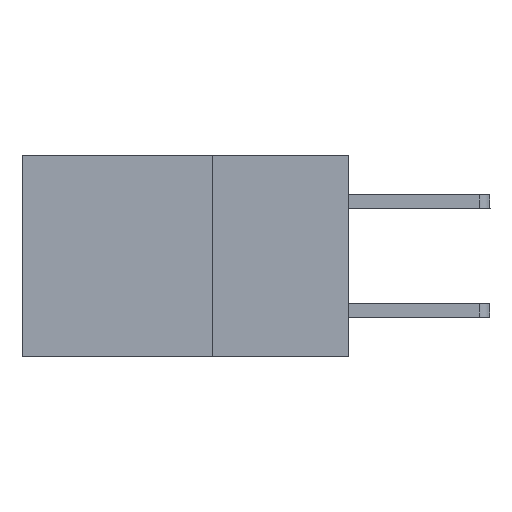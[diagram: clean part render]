
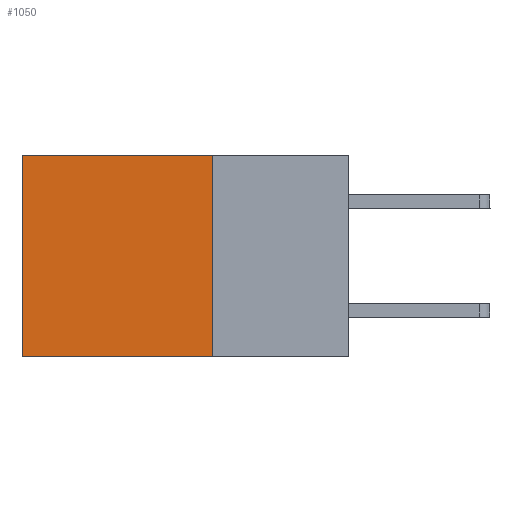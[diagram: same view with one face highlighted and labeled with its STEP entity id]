
A CAD part, left-side view. The second image highlights one B-rep face of the part: STEP entity #1050.
In plain terms, the highlighted planar face has unit normal (-1, 0, 0).
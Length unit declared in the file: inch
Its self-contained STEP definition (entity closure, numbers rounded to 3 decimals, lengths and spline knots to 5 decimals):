
#749 = VERTEX_POINT ( 'NONE', #8682 ) ;
#1047 = DIRECTION ( 'NONE',  ( 0., 0., -1. ) ) ;
#1050 = ADVANCED_FACE ( 'NONE', ( #9159 ), #6811, .F. ) ;
#1237 = CARTESIAN_POINT ( 'NONE',  ( 0.298, 0.25, 0. ) ) ;
#1526 = VECTOR ( 'NONE', #8058, 39.37008 ) ;
#1721 = CARTESIAN_POINT ( 'NONE',  ( 0.298, 0.25, 0. ) ) ;
#2336 = EDGE_LOOP ( 'NONE', ( #7548, #2485, #6023, #3111 ) ) ;
#2485 = ORIENTED_EDGE ( 'NONE', *, *, #5538, .F. ) ;
#2504 = AXIS2_PLACEMENT_3D ( 'NONE', #6103, #6990, #2613 ) ;
#2530 = VERTEX_POINT ( 'NONE', #4138 ) ;
#2613 = DIRECTION ( 'NONE',  ( 0., 0., -1. ) ) ;
#2627 = CARTESIAN_POINT ( 'NONE',  ( 0.298, 0.25, -0.37 ) ) ;
#3111 = ORIENTED_EDGE ( 'NONE', *, *, #6609, .T. ) ;
#3331 = VECTOR ( 'NONE', #1047, 39.37008 ) ;
#4132 = LINE ( 'NONE', #2627, #8996 ) ;
#4138 = CARTESIAN_POINT ( 'NONE',  ( 0.298, 0.6, 0. ) ) ;
#4605 = CARTESIAN_POINT ( 'NONE',  ( 0.298, 0.6, 0. ) ) ;
#5005 = LINE ( 'NONE', #7939, #7782 ) ;
#5076 = LINE ( 'NONE', #1721, #1526 ) ;
#5238 = VERTEX_POINT ( 'NONE', #1237 ) ;
#5538 = EDGE_CURVE ( 'NONE', #749, #7227, #4132, .T. ) ;
#6023 = ORIENTED_EDGE ( 'NONE', *, *, #7181, .F. ) ;
#6103 = CARTESIAN_POINT ( 'NONE',  ( 0.298, 0.25, 0. ) ) ;
#6609 = EDGE_CURVE ( 'NONE', #5238, #2530, #5005, .T. ) ;
#6811 = PLANE ( 'NONE',  #2504 ) ;
#6990 = DIRECTION ( 'NONE',  ( 1., 0., 0. ) ) ;
#7181 = EDGE_CURVE ( 'NONE', #5238, #749, #5076, .T. ) ;
#7227 = VERTEX_POINT ( 'NONE', #8020 ) ;
#7367 = EDGE_CURVE ( 'NONE', #2530, #7227, #8865, .T. ) ;
#7548 = ORIENTED_EDGE ( 'NONE', *, *, #7367, .T. ) ;
#7782 = VECTOR ( 'NONE', #8457, 39.37008 ) ;
#7939 = CARTESIAN_POINT ( 'NONE',  ( 0.298, 0.25, 0. ) ) ;
#8020 = CARTESIAN_POINT ( 'NONE',  ( 0.298, 0.6, -0.37 ) ) ;
#8058 = DIRECTION ( 'NONE',  ( 0., 0., -1. ) ) ;
#8315 = DIRECTION ( 'NONE',  ( 0., 1., 0. ) ) ;
#8457 = DIRECTION ( 'NONE',  ( 0., 1., 0. ) ) ;
#8682 = CARTESIAN_POINT ( 'NONE',  ( 0.298, 0.25, -0.37 ) ) ;
#8865 = LINE ( 'NONE', #4605, #3331 ) ;
#8996 = VECTOR ( 'NONE', #8315, 39.37008 ) ;
#9159 = FACE_OUTER_BOUND ( 'NONE', #2336, .T. ) ;
